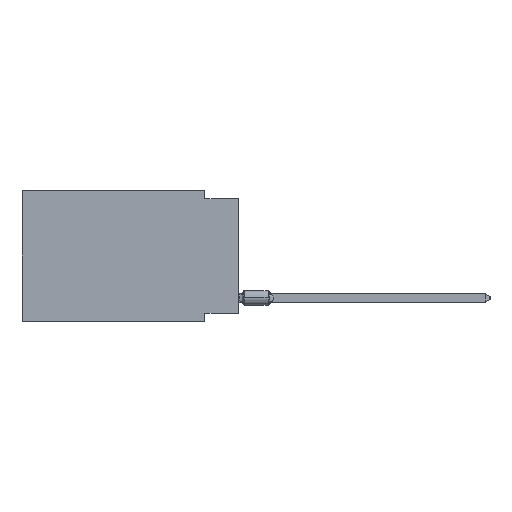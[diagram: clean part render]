
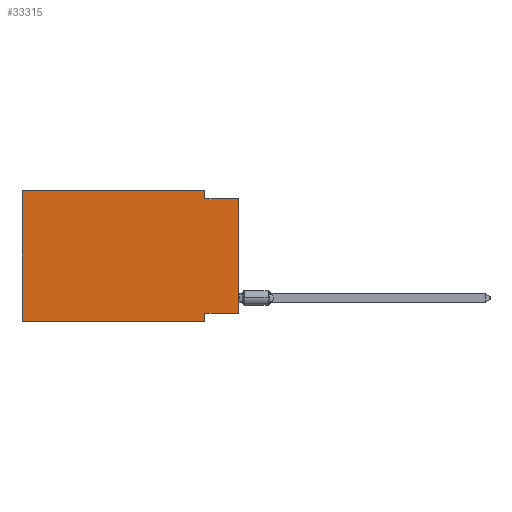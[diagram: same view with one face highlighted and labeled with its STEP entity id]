
A CAD part, left-side view. The second image highlights one B-rep face of the part: STEP entity #33315.
In plain terms, the highlighted planar face has unit normal (-1, 0, 0).
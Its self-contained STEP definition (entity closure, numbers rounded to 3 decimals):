
#837 = DIRECTION ( 'NONE',  ( 0., 0., 1. ) ) ;
#877 = CARTESIAN_POINT ( 'NONE',  ( 0., 16.383, -9.906 ) ) ;
#2769 = LINE ( 'NONE', #12307, #10984 ) ;
#2850 = ORIENTED_EDGE ( 'NONE', *, *, #25487, .F. ) ;
#3562 = VERTEX_POINT ( 'NONE', #26941 ) ;
#4087 = DIRECTION ( 'NONE',  ( 0., -1., 0. ) ) ;
#4876 = LINE ( 'NONE', #28068, #35088 ) ;
#7805 = VERTEX_POINT ( 'NONE', #25312 ) ;
#7880 = EDGE_CURVE ( 'NONE', #20916, #3562, #2769, .T. ) ;
#9168 = CARTESIAN_POINT ( 'NONE',  ( 0., 2.54, -0.635 ) ) ;
#9474 = PLANE ( 'NONE',  #18284 ) ;
#9881 = CARTESIAN_POINT ( 'NONE',  ( 0., 2.54, -9.271 ) ) ;
#10548 = CARTESIAN_POINT ( 'NONE',  ( 0., 2.54, -9.906 ) ) ;
#10665 = ORIENTED_EDGE ( 'NONE', *, *, #12951, .F. ) ;
#10685 = VECTOR ( 'NONE', #24476, 1000. ) ;
#10887 = ORIENTED_EDGE ( 'NONE', *, *, #42901, .F. ) ;
#10984 = VECTOR ( 'NONE', #42708, 1000. ) ;
#11791 = CARTESIAN_POINT ( 'NONE',  ( 0., 16.383, 0. ) ) ;
#12212 = VERTEX_POINT ( 'NONE', #9881 ) ;
#12307 = CARTESIAN_POINT ( 'NONE',  ( 0., 16.383, -9.906 ) ) ;
#12753 = ORIENTED_EDGE ( 'NONE', *, *, #41777, .T. ) ;
#12951 = EDGE_CURVE ( 'NONE', #39275, #41770, #18857, .T. ) ;
#13585 = ORIENTED_EDGE ( 'NONE', *, *, #7880, .T. ) ;
#13893 = DIRECTION ( 'NONE',  ( 0., 0., -1. ) ) ;
#14338 = LINE ( 'NONE', #33666, #14811 ) ;
#14811 = VECTOR ( 'NONE', #27561, 1000. ) ;
#16122 = EDGE_LOOP ( 'NONE', ( #12753, #24375, #19338, #10665, #29367, #13585, #10887, #2850 ) ) ;
#16424 = DIRECTION ( 'NONE',  ( 0., 0., -1. ) ) ;
#17524 = CARTESIAN_POINT ( 'NONE',  ( 0., 16.383, 0. ) ) ;
#18284 = AXIS2_PLACEMENT_3D ( 'NONE', #22943, #28793, #16424 ) ;
#18857 = LINE ( 'NONE', #24030, #42494 ) ;
#19041 = FACE_OUTER_BOUND ( 'NONE', #16122, .T. ) ;
#19338 = ORIENTED_EDGE ( 'NONE', *, *, #22649, .F. ) ;
#20141 = LINE ( 'NONE', #17524, #35809 ) ;
#20916 = VERTEX_POINT ( 'NONE', #877 ) ;
#22649 = EDGE_CURVE ( 'NONE', #41770, #40685, #23239, .T. ) ;
#22943 = CARTESIAN_POINT ( 'NONE',  ( 0., 16.383, 0. ) ) ;
#23239 = LINE ( 'NONE', #27124, #39910 ) ;
#23485 = EDGE_CURVE ( 'NONE', #20916, #39275, #20141, .T. ) ;
#24030 = CARTESIAN_POINT ( 'NONE',  ( 0., 16.383, 0. ) ) ;
#24375 = ORIENTED_EDGE ( 'NONE', *, *, #31318, .F. ) ;
#24476 = DIRECTION ( 'NONE',  ( 0., 1., 0. ) ) ;
#25312 = CARTESIAN_POINT ( 'NONE',  ( 0., 0., -0.635 ) ) ;
#25487 = EDGE_CURVE ( 'NONE', #39763, #12212, #27737, .T. ) ;
#26941 = CARTESIAN_POINT ( 'NONE',  ( 0., 2.54, -9.906 ) ) ;
#27124 = CARTESIAN_POINT ( 'NONE',  ( 0., 2.54, 0. ) ) ;
#27310 = CARTESIAN_POINT ( 'NONE',  ( 0., 0., -9.271 ) ) ;
#27561 = DIRECTION ( 'NONE',  ( 0., -1., 0. ) ) ;
#27737 = LINE ( 'NONE', #27310, #10685 ) ;
#27866 = DIRECTION ( 'NONE',  ( 0., 0., 1. ) ) ;
#28068 = CARTESIAN_POINT ( 'NONE',  ( 0., 0., 0. ) ) ;
#28793 = DIRECTION ( 'NONE',  ( 1., 0., 0. ) ) ;
#29367 = ORIENTED_EDGE ( 'NONE', *, *, #23485, .F. ) ;
#31318 = EDGE_CURVE ( 'NONE', #40685, #7805, #14338, .T. ) ;
#33315 = ADVANCED_FACE ( 'NONE', ( #19041 ), #9474, .F. ) ;
#33336 = LINE ( 'NONE', #10548, #37933 ) ;
#33666 = CARTESIAN_POINT ( 'NONE',  ( 0., 0., -0.635 ) ) ;
#35088 = VECTOR ( 'NONE', #27866, 1000. ) ;
#35809 = VECTOR ( 'NONE', #837, 1000. ) ;
#35814 = CARTESIAN_POINT ( 'NONE',  ( 0., 0., -9.271 ) ) ;
#37242 = DIRECTION ( 'NONE',  ( 0., 0., -1. ) ) ;
#37933 = VECTOR ( 'NONE', #37242, 1000. ) ;
#38072 = CARTESIAN_POINT ( 'NONE',  ( 0., 2.54, 0. ) ) ;
#39275 = VERTEX_POINT ( 'NONE', #11791 ) ;
#39763 = VERTEX_POINT ( 'NONE', #35814 ) ;
#39910 = VECTOR ( 'NONE', #13893, 1000. ) ;
#40685 = VERTEX_POINT ( 'NONE', #9168 ) ;
#41770 = VERTEX_POINT ( 'NONE', #38072 ) ;
#41777 = EDGE_CURVE ( 'NONE', #39763, #7805, #4876, .T. ) ;
#42494 = VECTOR ( 'NONE', #4087, 1000. ) ;
#42708 = DIRECTION ( 'NONE',  ( 0., -1., 0. ) ) ;
#42901 = EDGE_CURVE ( 'NONE', #12212, #3562, #33336, .T. ) ;
